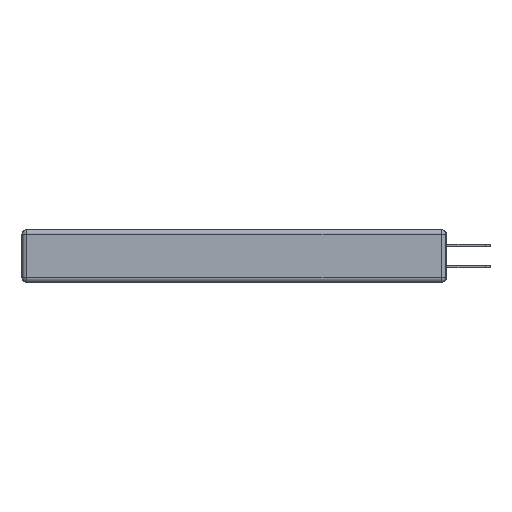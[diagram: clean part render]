
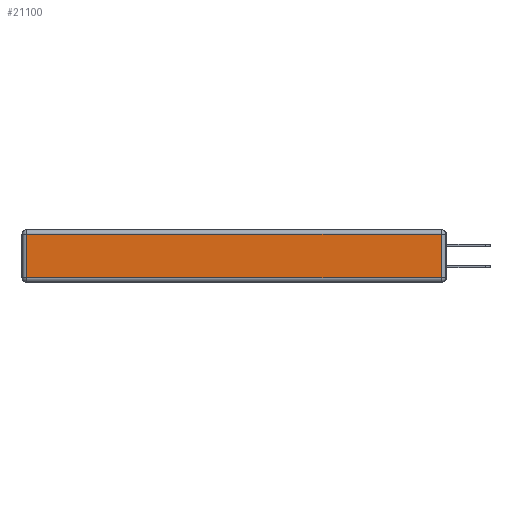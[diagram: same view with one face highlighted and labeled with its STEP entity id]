
A CAD part, left-side view. The second image highlights one B-rep face of the part: STEP entity #21100.
In plain terms, the highlighted planar face has unit normal (-1, 0, 0).
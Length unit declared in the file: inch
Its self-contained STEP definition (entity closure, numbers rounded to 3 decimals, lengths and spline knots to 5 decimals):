
#190 = CARTESIAN_POINT ( 'NONE',  ( 0., 0.03, -0.313 ) ) ;
#721 = ORIENTED_EDGE ( 'NONE', *, *, #11139, .T. ) ;
#1797 = EDGE_CURVE ( 'NONE', #22112, #16817, #6543, .T. ) ;
#2634 = CARTESIAN_POINT ( 'NONE',  ( 0., 2.72, -0.313 ) ) ;
#3790 = ORIENTED_EDGE ( 'NONE', *, *, #10222, .T. ) ;
#5138 = ORIENTED_EDGE ( 'NONE', *, *, #1797, .T. ) ;
#5545 = CARTESIAN_POINT ( 'NONE',  ( 0., 2.75, -0.03 ) ) ;
#5915 = DIRECTION ( 'NONE',  ( 0., -1., 0. ) ) ;
#6065 = CARTESIAN_POINT ( 'NONE',  ( 0., 0., -0.313 ) ) ;
#6543 = LINE ( 'NONE', #5545, #11214 ) ;
#6553 = DIRECTION ( 'NONE',  ( 0., 0., 1. ) ) ;
#7072 = CARTESIAN_POINT ( 'NONE',  ( 0., 0.03, -0.03 ) ) ;
#7362 = LINE ( 'NONE', #20329, #17610 ) ;
#7712 = VECTOR ( 'NONE', #5915, 39.37008 ) ;
#8683 = FACE_OUTER_BOUND ( 'NONE', #20447, .T. ) ;
#10222 = EDGE_CURVE ( 'NONE', #19249, #15284, #11228, .T. ) ;
#11139 = EDGE_CURVE ( 'NONE', #16817, #19249, #7362, .T. ) ;
#11214 = VECTOR ( 'NONE', #13484, 39.37008 ) ;
#11228 = LINE ( 'NONE', #6065, #7712 ) ;
#11394 = ORIENTED_EDGE ( 'NONE', *, *, #23524, .T. ) ;
#12222 = DIRECTION ( 'NONE',  ( 0., 0., 1. ) ) ;
#13484 = DIRECTION ( 'NONE',  ( 0., 1., 0. ) ) ;
#14112 = CARTESIAN_POINT ( 'NONE',  ( 0., 0., -0.343 ) ) ;
#15000 = VECTOR ( 'NONE', #6553, 39.37008 ) ;
#15284 = VERTEX_POINT ( 'NONE', #190 ) ;
#16631 = DIRECTION ( 'NONE',  ( 0., 0., -1. ) ) ;
#16731 = CARTESIAN_POINT ( 'NONE',  ( 0., 2.72, -0.03 ) ) ;
#16817 = VERTEX_POINT ( 'NONE', #16731 ) ;
#17421 = CARTESIAN_POINT ( 'NONE',  ( 0., 0.03, -0.343 ) ) ;
#17610 = VECTOR ( 'NONE', #16631, 39.37008 ) ;
#19094 = LINE ( 'NONE', #17421, #15000 ) ;
#19249 = VERTEX_POINT ( 'NONE', #2634 ) ;
#20329 = CARTESIAN_POINT ( 'NONE',  ( 0., 2.72, -0.343 ) ) ;
#20402 = AXIS2_PLACEMENT_3D ( 'NONE', #14112, #23363, #12222 ) ;
#20447 = EDGE_LOOP ( 'NONE', ( #3790, #11394, #5138, #721 ) ) ;
#21100 = ADVANCED_FACE ( 'NONE', ( #8683 ), #21739, .T. ) ;
#21739 = PLANE ( 'NONE',  #20402 ) ;
#22112 = VERTEX_POINT ( 'NONE', #7072 ) ;
#23363 = DIRECTION ( 'NONE',  ( -1., 0., 0. ) ) ;
#23524 = EDGE_CURVE ( 'NONE', #15284, #22112, #19094, .T. ) ;
